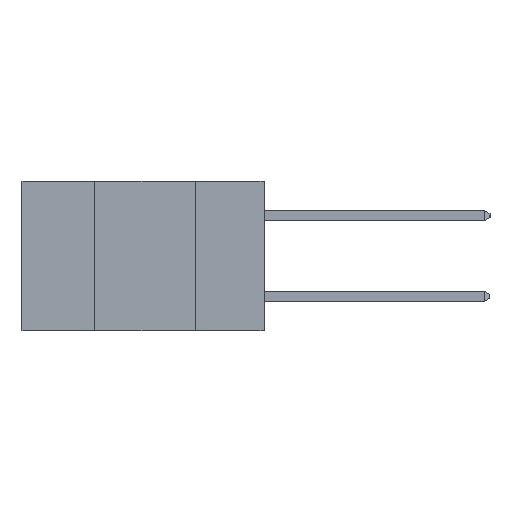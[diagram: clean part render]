
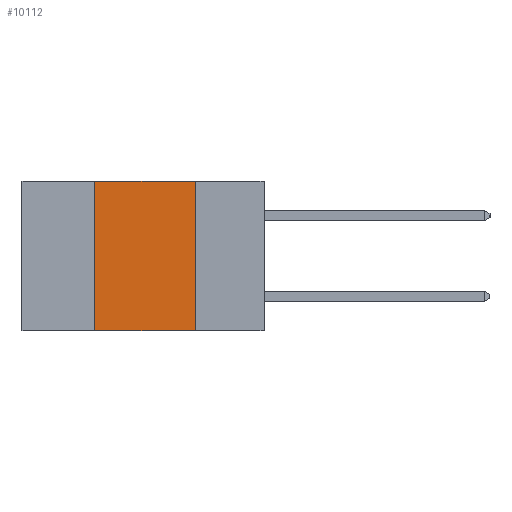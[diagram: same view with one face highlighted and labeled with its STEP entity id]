
A CAD part, left-side view. The second image highlights one B-rep face of the part: STEP entity #10112.
In plain terms, the highlighted planar face has unit normal (-1, 0, 0).
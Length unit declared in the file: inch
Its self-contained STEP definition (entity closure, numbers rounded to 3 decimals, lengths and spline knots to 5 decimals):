
#2 = DIRECTION ( 'NONE',  ( 0., 0., -1. ) ) ;
#19 = LINE ( 'NONE', #10572, #2816 ) ;
#1029 = DIRECTION ( 'NONE',  ( 1., 0., 0. ) ) ;
#1260 = EDGE_CURVE ( 'NONE', #6023, #12160, #19, .T. ) ;
#1820 = VECTOR ( 'NONE', #8959, 39.37008 ) ;
#1863 = ORIENTED_EDGE ( 'NONE', *, *, #12037, .T. ) ;
#2513 = ORIENTED_EDGE ( 'NONE', *, *, #1260, .F. ) ;
#2816 = VECTOR ( 'NONE', #3790, 39.37008 ) ;
#3341 = EDGE_CURVE ( 'NONE', #7067, #6803, #7273, .T. ) ;
#3614 = LINE ( 'NONE', #11753, #5971 ) ;
#3790 = DIRECTION ( 'NONE',  ( 0., 0., 1. ) ) ;
#3807 = CARTESIAN_POINT ( 'NONE',  ( 0., 0.17, -0.37 ) ) ;
#4242 = EDGE_LOOP ( 'NONE', ( #11996, #9499, #2513, #1863 ) ) ;
#5043 = CARTESIAN_POINT ( 'NONE',  ( 0., 0.6, 0. ) ) ;
#5971 = VECTOR ( 'NONE', #12606, 39.37008 ) ;
#6023 = VERTEX_POINT ( 'NONE', #6643 ) ;
#6575 = CARTESIAN_POINT ( 'NONE',  ( 0., 0.17, 0. ) ) ;
#6643 = CARTESIAN_POINT ( 'NONE',  ( 0., 0.42, -0.37 ) ) ;
#6803 = VERTEX_POINT ( 'NONE', #3807 ) ;
#7067 = VERTEX_POINT ( 'NONE', #9128 ) ;
#7273 = LINE ( 'NONE', #6575, #12046 ) ;
#8052 = DIRECTION ( 'NONE',  ( 0., 0., -1. ) ) ;
#8959 = DIRECTION ( 'NONE',  ( 0., -1., 0. ) ) ;
#9128 = CARTESIAN_POINT ( 'NONE',  ( 0., 0.17, 0. ) ) ;
#9442 = EDGE_CURVE ( 'NONE', #12160, #7067, #12215, .T. ) ;
#9499 = ORIENTED_EDGE ( 'NONE', *, *, #9442, .F. ) ;
#10043 = CARTESIAN_POINT ( 'NONE',  ( 0., 0.42, 0. ) ) ;
#10112 = ADVANCED_FACE ( 'NONE', ( #11796 ), #12702, .F. ) ;
#10236 = AXIS2_PLACEMENT_3D ( 'NONE', #10945, #1029, #8052 ) ;
#10572 = CARTESIAN_POINT ( 'NONE',  ( 0., 0.42, 0. ) ) ;
#10945 = CARTESIAN_POINT ( 'NONE',  ( 0., 0.6, 0. ) ) ;
#11753 = CARTESIAN_POINT ( 'NONE',  ( 0., 0.6, -0.37 ) ) ;
#11796 = FACE_OUTER_BOUND ( 'NONE', #4242, .T. ) ;
#11996 = ORIENTED_EDGE ( 'NONE', *, *, #3341, .F. ) ;
#12037 = EDGE_CURVE ( 'NONE', #6023, #6803, #3614, .T. ) ;
#12046 = VECTOR ( 'NONE', #2, 39.37008 ) ;
#12160 = VERTEX_POINT ( 'NONE', #10043 ) ;
#12215 = LINE ( 'NONE', #5043, #1820 ) ;
#12606 = DIRECTION ( 'NONE',  ( 0., -1., 0. ) ) ;
#12702 = PLANE ( 'NONE',  #10236 ) ;
